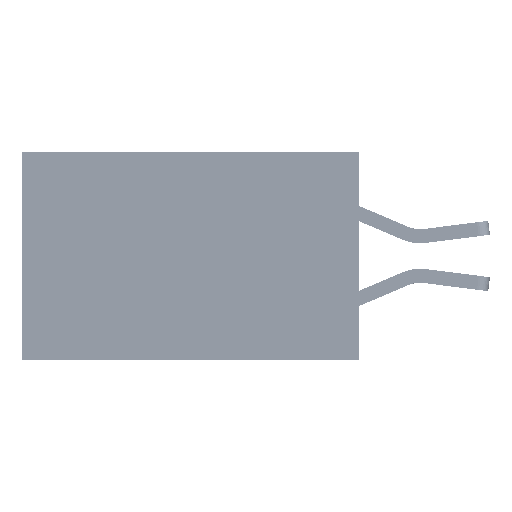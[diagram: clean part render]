
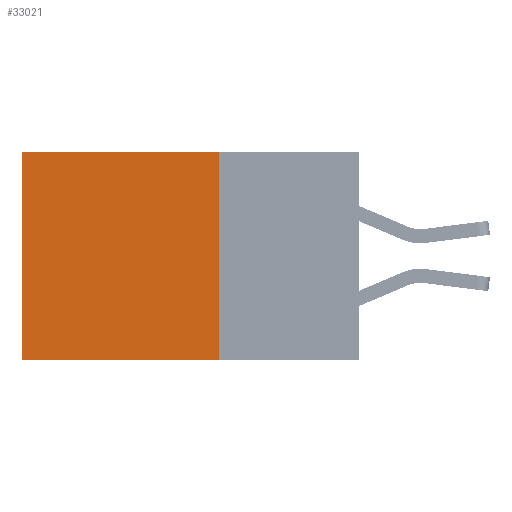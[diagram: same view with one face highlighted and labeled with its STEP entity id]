
A CAD part, left-side view. The second image highlights one B-rep face of the part: STEP entity #33021.
In plain terms, the highlighted planar face has unit normal (-1, 0, 0).
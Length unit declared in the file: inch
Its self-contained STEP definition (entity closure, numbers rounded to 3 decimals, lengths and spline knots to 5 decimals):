
#1843 = ORIENTED_EDGE ( 'NONE', *, *, #25284, .T. ) ;
#2749 = LINE ( 'NONE', #25571, #15236 ) ;
#3303 = VERTEX_POINT ( 'NONE', #13669 ) ;
#3509 = LINE ( 'NONE', #31286, #37230 ) ;
#6397 = VECTOR ( 'NONE', #40295, 39.37008 ) ;
#9995 = ORIENTED_EDGE ( 'NONE', *, *, #13278, .T. ) ;
#10278 = VERTEX_POINT ( 'NONE', #26304 ) ;
#11250 = ORIENTED_EDGE ( 'NONE', *, *, #35846, .F. ) ;
#11423 = CARTESIAN_POINT ( 'NONE',  ( 0.2875, 0.25, -0.37 ) ) ;
#13278 = EDGE_CURVE ( 'NONE', #3303, #10278, #2749, .T. ) ;
#13323 = PLANE ( 'NONE',  #21214 ) ;
#13669 = CARTESIAN_POINT ( 'NONE',  ( 0.2875, 0.6, 0. ) ) ;
#15236 = VECTOR ( 'NONE', #34851, 39.37008 ) ;
#15538 = DIRECTION ( 'NONE',  ( 0., 1., 0. ) ) ;
#16782 = DIRECTION ( 'NONE',  ( 1., 0., 0. ) ) ;
#17600 = FACE_OUTER_BOUND ( 'NONE', #20109, .T. ) ;
#19895 = ORIENTED_EDGE ( 'NONE', *, *, #29923, .F. ) ;
#20109 = EDGE_LOOP ( 'NONE', ( #9995, #11250, #19895, #1843 ) ) ;
#21214 = AXIS2_PLACEMENT_3D ( 'NONE', #35434, #16782, #29739 ) ;
#21679 = VECTOR ( 'NONE', #40832, 39.37008 ) ;
#25284 = EDGE_CURVE ( 'NONE', #31371, #3303, #3509, .T. ) ;
#25571 = CARTESIAN_POINT ( 'NONE',  ( 0.2875, 0.6, 0. ) ) ;
#26304 = CARTESIAN_POINT ( 'NONE',  ( 0.2875, 0.6, -0.37 ) ) ;
#28579 = LINE ( 'NONE', #11423, #21679 ) ;
#28626 = CARTESIAN_POINT ( 'NONE',  ( 0.2875, 0.25, -0.37 ) ) ;
#28670 = LINE ( 'NONE', #33910, #6397 ) ;
#29613 = VERTEX_POINT ( 'NONE', #28626 ) ;
#29739 = DIRECTION ( 'NONE',  ( 0., 0., -1. ) ) ;
#29923 = EDGE_CURVE ( 'NONE', #31371, #29613, #28670, .T. ) ;
#31286 = CARTESIAN_POINT ( 'NONE',  ( 0.2875, 0.25, 0. ) ) ;
#31371 = VERTEX_POINT ( 'NONE', #36843 ) ;
#33021 = ADVANCED_FACE ( 'NONE', ( #17600 ), #13323, .F. ) ;
#33910 = CARTESIAN_POINT ( 'NONE',  ( 0.2875, 0.25, 0. ) ) ;
#34851 = DIRECTION ( 'NONE',  ( 0., 0., -1. ) ) ;
#35434 = CARTESIAN_POINT ( 'NONE',  ( 0.2875, 0.25, 0. ) ) ;
#35846 = EDGE_CURVE ( 'NONE', #29613, #10278, #28579, .T. ) ;
#36843 = CARTESIAN_POINT ( 'NONE',  ( 0.2875, 0.25, 0. ) ) ;
#37230 = VECTOR ( 'NONE', #15538, 39.37008 ) ;
#40295 = DIRECTION ( 'NONE',  ( 0., 0., -1. ) ) ;
#40832 = DIRECTION ( 'NONE',  ( 0., 1., 0. ) ) ;
